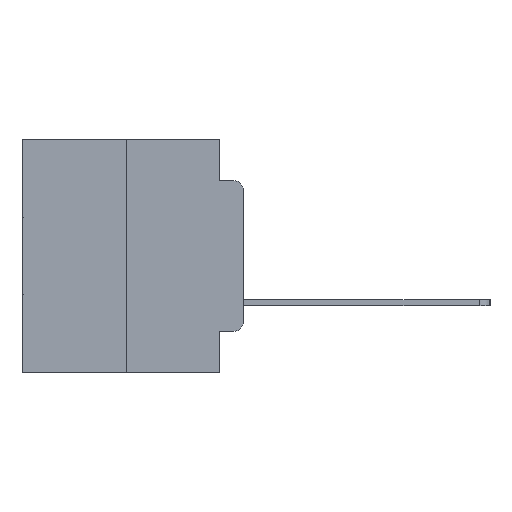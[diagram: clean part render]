
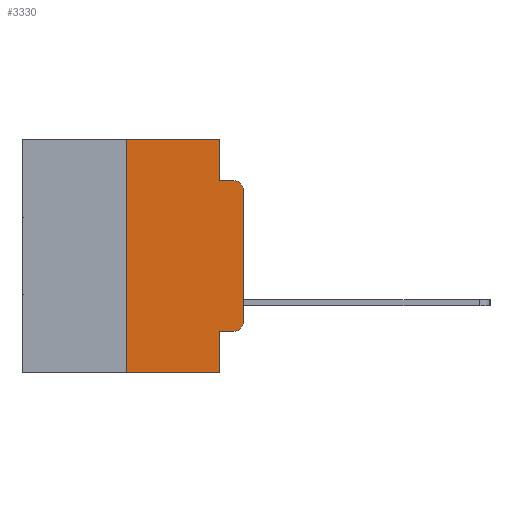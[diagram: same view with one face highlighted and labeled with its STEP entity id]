
A CAD part, left-side view. The second image highlights one B-rep face of the part: STEP entity #3330.
In plain terms, the highlighted planar face has unit normal (-1, 0, 0).
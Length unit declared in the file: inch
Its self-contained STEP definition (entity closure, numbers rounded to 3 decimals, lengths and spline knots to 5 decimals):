
#800 = ORIENTED_EDGE ( 'NONE', *, *, #2890, .F. ) ;
#1074 = DIRECTION ( 'NONE',  ( -1., 0., 0. ) ) ;
#1358 = EDGE_CURVE ( 'NONE', #11330, #7917, #15198, .T. ) ;
#2345 = AXIS2_PLACEMENT_3D ( 'NONE', #25364, #11127, #27538 ) ;
#2536 = DIRECTION ( 'NONE',  ( 0., -1., 0. ) ) ;
#2687 = CARTESIAN_POINT ( 'NONE',  ( 0., 0.051, -0.4115 ) ) ;
#2890 = EDGE_CURVE ( 'NONE', #7917, #7564, #27244, .T. ) ;
#3325 = CARTESIAN_POINT ( 'NONE',  ( 0., 0., -0.3915 ) ) ;
#3330 = ADVANCED_FACE ( 'NONE', ( #14791 ), #21667, .F. ) ;
#3530 = CARTESIAN_POINT ( 'NONE',  ( 0., 0.25, 0. ) ) ;
#4031 = VERTEX_POINT ( 'NONE', #20099 ) ;
#4455 = EDGE_CURVE ( 'NONE', #4031, #7564, #8724, .T. ) ;
#4632 = LINE ( 'NONE', #24991, #22072 ) ;
#5770 = AXIS2_PLACEMENT_3D ( 'NONE', #23068, #8806, #25345 ) ;
#6050 = EDGE_CURVE ( 'NONE', #20324, #4031, #18717, .T. ) ;
#7510 = DIRECTION ( 'NONE',  ( 0., 0., -1. ) ) ;
#7564 = VERTEX_POINT ( 'NONE', #28100 ) ;
#7789 = DIRECTION ( 'NONE',  ( 0., 0., 1. ) ) ;
#7917 = VERTEX_POINT ( 'NONE', #8499 ) ;
#8103 = DIRECTION ( 'NONE',  ( 0., 0., 1. ) ) ;
#8499 = CARTESIAN_POINT ( 'NONE',  ( 0., 0.051, -0.0885 ) ) ;
#8724 = CIRCLE ( 'NONE', #11587, 0.02 ) ;
#8806 = DIRECTION ( 'NONE',  ( -1., 0., 0. ) ) ;
#8904 = ORIENTED_EDGE ( 'NONE', *, *, #6050, .T. ) ;
#9282 = LINE ( 'NONE', #3530, #14917 ) ;
#9318 = LINE ( 'NONE', #23757, #21264 ) ;
#11080 = CARTESIAN_POINT ( 'NONE',  ( 0., 0.051, -0.5 ) ) ;
#11127 = DIRECTION ( 'NONE',  ( 1., 0., 0. ) ) ;
#11330 = VERTEX_POINT ( 'NONE', #22395 ) ;
#11587 = AXIS2_PLACEMENT_3D ( 'NONE', #15184, #1074, #13170 ) ;
#11722 = VERTEX_POINT ( 'NONE', #2687 ) ;
#12079 = ORIENTED_EDGE ( 'NONE', *, *, #30083, .F. ) ;
#13170 = DIRECTION ( 'NONE',  ( 0., 0., -1. ) ) ;
#13265 = VECTOR ( 'NONE', #24518, 39.37008 ) ;
#14328 = DIRECTION ( 'NONE',  ( 0., 0., -1. ) ) ;
#14791 = FACE_OUTER_BOUND ( 'NONE', #21059, .T. ) ;
#14917 = VECTOR ( 'NONE', #8103, 39.37008 ) ;
#15184 = CARTESIAN_POINT ( 'NONE',  ( 0., 0.02, -0.1085 ) ) ;
#15198 = LINE ( 'NONE', #23292, #22271 ) ;
#15435 = ORIENTED_EDGE ( 'NONE', *, *, #28577, .F. ) ;
#15959 = LINE ( 'NONE', #16598, #22281 ) ;
#16598 = CARTESIAN_POINT ( 'NONE',  ( 0., 0.473, 0. ) ) ;
#17762 = CARTESIAN_POINT ( 'NONE',  ( 0., 0.25, 0. ) ) ;
#18717 = LINE ( 'NONE', #24368, #19477 ) ;
#18794 = VERTEX_POINT ( 'NONE', #22378 ) ;
#19477 = VECTOR ( 'NONE', #7789, 39.37008 ) ;
#19719 = VERTEX_POINT ( 'NONE', #17762 ) ;
#19777 = EDGE_CURVE ( 'NONE', #18794, #22793, #4632, .T. ) ;
#19826 = CARTESIAN_POINT ( 'NONE',  ( 0., 0.051, -0.4115 ) ) ;
#20007 = ORIENTED_EDGE ( 'NONE', *, *, #24848, .F. ) ;
#20076 = ORIENTED_EDGE ( 'NONE', *, *, #4455, .T. ) ;
#20099 = CARTESIAN_POINT ( 'NONE',  ( 0., 0., -0.1085 ) ) ;
#20324 = VERTEX_POINT ( 'NONE', #3325 ) ;
#20384 = CARTESIAN_POINT ( 'NONE',  ( 0., 0.02, -0.4115 ) ) ;
#20387 = LINE ( 'NONE', #19826, #13265 ) ;
#20425 = VECTOR ( 'NONE', #26799, 39.37008 ) ;
#21059 = EDGE_LOOP ( 'NONE', ( #8904, #20076, #800, #28650, #20007, #12079, #29055, #15435, #21258, #29912 ) ) ;
#21258 = ORIENTED_EDGE ( 'NONE', *, *, #25564, .T. ) ;
#21264 = VECTOR ( 'NONE', #14328, 39.37008 ) ;
#21667 = PLANE ( 'NONE',  #2345 ) ;
#22072 = VECTOR ( 'NONE', #29508, 39.37008 ) ;
#22271 = VECTOR ( 'NONE', #7510, 39.37008 ) ;
#22281 = VECTOR ( 'NONE', #2536, 39.37008 ) ;
#22329 = CARTESIAN_POINT ( 'NONE',  ( 0., 0.051, -0.0885 ) ) ;
#22378 = CARTESIAN_POINT ( 'NONE',  ( 0., 0.25, -0.5 ) ) ;
#22395 = CARTESIAN_POINT ( 'NONE',  ( 0., 0.051, 0. ) ) ;
#22793 = VERTEX_POINT ( 'NONE', #11080 ) ;
#23068 = CARTESIAN_POINT ( 'NONE',  ( 0., 0.02, -0.3915 ) ) ;
#23292 = CARTESIAN_POINT ( 'NONE',  ( 0., 0.051, 0. ) ) ;
#23757 = CARTESIAN_POINT ( 'NONE',  ( 0., 0.051, 0. ) ) ;
#24061 = EDGE_CURVE ( 'NONE', #24565, #20324, #26241, .T. ) ;
#24368 = CARTESIAN_POINT ( 'NONE',  ( 0., 0., 0. ) ) ;
#24518 = DIRECTION ( 'NONE',  ( 0., -1., 0. ) ) ;
#24565 = VERTEX_POINT ( 'NONE', #20384 ) ;
#24848 = EDGE_CURVE ( 'NONE', #19719, #11330, #15959, .T. ) ;
#24991 = CARTESIAN_POINT ( 'NONE',  ( 0., 0.473, -0.5 ) ) ;
#25345 = DIRECTION ( 'NONE',  ( 0., 0., -1. ) ) ;
#25364 = CARTESIAN_POINT ( 'NONE',  ( 0., 0.473, 0. ) ) ;
#25564 = EDGE_CURVE ( 'NONE', #11722, #24565, #20387, .T. ) ;
#26241 = CIRCLE ( 'NONE', #5770, 0.02 ) ;
#26799 = DIRECTION ( 'NONE',  ( 0., -1., 0. ) ) ;
#27244 = LINE ( 'NONE', #22329, #20425 ) ;
#27538 = DIRECTION ( 'NONE',  ( 0., 0., -1. ) ) ;
#28100 = CARTESIAN_POINT ( 'NONE',  ( 0., 0.02, -0.0885 ) ) ;
#28577 = EDGE_CURVE ( 'NONE', #11722, #22793, #9318, .T. ) ;
#28650 = ORIENTED_EDGE ( 'NONE', *, *, #1358, .F. ) ;
#29055 = ORIENTED_EDGE ( 'NONE', *, *, #19777, .T. ) ;
#29508 = DIRECTION ( 'NONE',  ( 0., -1., 0. ) ) ;
#29912 = ORIENTED_EDGE ( 'NONE', *, *, #24061, .T. ) ;
#30083 = EDGE_CURVE ( 'NONE', #18794, #19719, #9282, .T. ) ;
